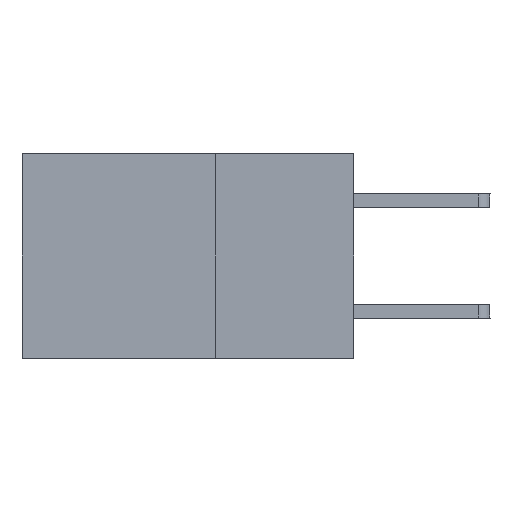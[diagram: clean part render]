
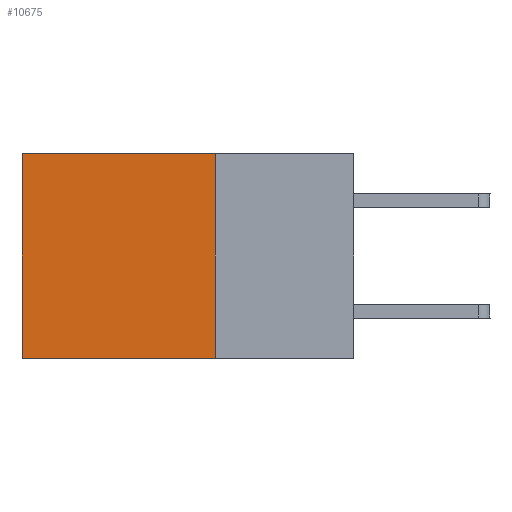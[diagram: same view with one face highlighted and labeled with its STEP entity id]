
A CAD part, left-side view. The second image highlights one B-rep face of the part: STEP entity #10675.
In plain terms, the highlighted planar face has unit normal (-1, 0, 0).
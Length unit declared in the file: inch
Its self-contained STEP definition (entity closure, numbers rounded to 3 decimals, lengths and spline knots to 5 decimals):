
#112 = CARTESIAN_POINT ( 'NONE',  ( 0.2875, 0.25, -0.37 ) ) ;
#594 = LINE ( 'NONE', #12952, #9630 ) ;
#675 = LINE ( 'NONE', #10555, #7101 ) ;
#720 = ORIENTED_EDGE ( 'NONE', *, *, #7247, .F. ) ;
#1069 = CARTESIAN_POINT ( 'NONE',  ( 0.2875, 0.25, 0. ) ) ;
#1364 = DIRECTION ( 'NONE',  ( 1., 0., 0. ) ) ;
#1752 = VECTOR ( 'NONE', #9183, 39.37008 ) ;
#1973 = EDGE_LOOP ( 'NONE', ( #9541, #3657, #720, #3509 ) ) ;
#2087 = CARTESIAN_POINT ( 'NONE',  ( 0.2875, 0.6, -0.37 ) ) ;
#2377 = LINE ( 'NONE', #1069, #8426 ) ;
#2580 = EDGE_CURVE ( 'NONE', #11170, #3456, #675, .T. ) ;
#3456 = VERTEX_POINT ( 'NONE', #2087 ) ;
#3509 = ORIENTED_EDGE ( 'NONE', *, *, #9232, .T. ) ;
#3550 = PLANE ( 'NONE',  #14318 ) ;
#3657 = ORIENTED_EDGE ( 'NONE', *, *, #13746, .F. ) ;
#4049 = DIRECTION ( 'NONE',  ( 0., 0., -1. ) ) ;
#4708 = CARTESIAN_POINT ( 'NONE',  ( 0.2875, 0.25, -0.37 ) ) ;
#4986 = CARTESIAN_POINT ( 'NONE',  ( 0.2875, 0.25, 0. ) ) ;
#5538 = DIRECTION ( 'NONE',  ( 0., 0., -1. ) ) ;
#5859 = CARTESIAN_POINT ( 'NONE',  ( 0.2875, 0.6, 0. ) ) ;
#6723 = VERTEX_POINT ( 'NONE', #4986 ) ;
#7101 = VECTOR ( 'NONE', #4049, 39.37008 ) ;
#7247 = EDGE_CURVE ( 'NONE', #6723, #10593, #2377, .T. ) ;
#7392 = DIRECTION ( 'NONE',  ( 0., 1., 0. ) ) ;
#8167 = CARTESIAN_POINT ( 'NONE',  ( 0.2875, 0.25, 0. ) ) ;
#8227 = LINE ( 'NONE', #4708, #1752 ) ;
#8426 = VECTOR ( 'NONE', #5538, 39.37008 ) ;
#9120 = DIRECTION ( 'NONE',  ( 0., 0., -1. ) ) ;
#9183 = DIRECTION ( 'NONE',  ( 0., 1., 0. ) ) ;
#9232 = EDGE_CURVE ( 'NONE', #6723, #11170, #594, .T. ) ;
#9541 = ORIENTED_EDGE ( 'NONE', *, *, #2580, .T. ) ;
#9630 = VECTOR ( 'NONE', #7392, 39.37008 ) ;
#10356 = FACE_OUTER_BOUND ( 'NONE', #1973, .T. ) ;
#10555 = CARTESIAN_POINT ( 'NONE',  ( 0.2875, 0.6, 0. ) ) ;
#10593 = VERTEX_POINT ( 'NONE', #112 ) ;
#10675 = ADVANCED_FACE ( 'NONE', ( #10356 ), #3550, .F. ) ;
#11170 = VERTEX_POINT ( 'NONE', #5859 ) ;
#12952 = CARTESIAN_POINT ( 'NONE',  ( 0.2875, 0.25, 0. ) ) ;
#13746 = EDGE_CURVE ( 'NONE', #10593, #3456, #8227, .T. ) ;
#14318 = AXIS2_PLACEMENT_3D ( 'NONE', #8167, #1364, #9120 ) ;
